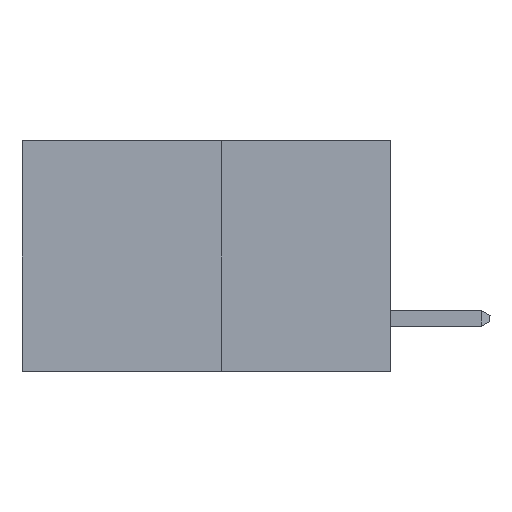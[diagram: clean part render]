
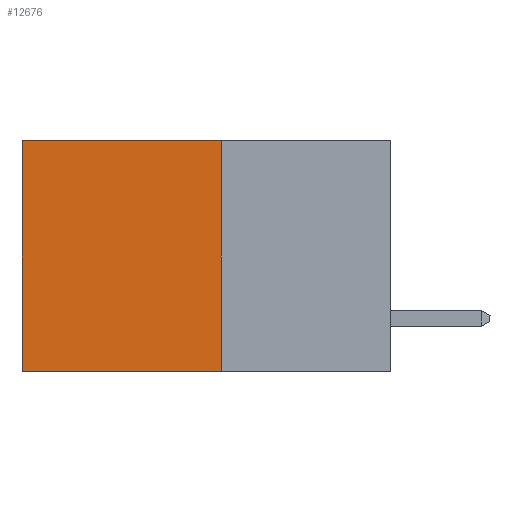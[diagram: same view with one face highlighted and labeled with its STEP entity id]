
A CAD part, left-side view. The second image highlights one B-rep face of the part: STEP entity #12676.
In plain terms, the highlighted planar face has unit normal (-1, 0, 0).
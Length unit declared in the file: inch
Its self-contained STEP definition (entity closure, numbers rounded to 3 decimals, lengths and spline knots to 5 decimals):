
#1009 = CARTESIAN_POINT ( 'NONE',  ( 0.277, 0.59, -0.37 ) ) ;
#1265 = VECTOR ( 'NONE', #9270, 39.37008 ) ;
#1685 = ORIENTED_EDGE ( 'NONE', *, *, #2820, .F. ) ;
#2820 = EDGE_CURVE ( 'NONE', #13778, #4900, #4460, .T. ) ;
#2873 = CARTESIAN_POINT ( 'NONE',  ( 0.277, 0.27, -0.37 ) ) ;
#2980 = DIRECTION ( 'NONE',  ( 0., 0., -1. ) ) ;
#3701 = LINE ( 'NONE', #12434, #9588 ) ;
#4460 = LINE ( 'NONE', #13301, #1265 ) ;
#4637 = EDGE_CURVE ( 'NONE', #13310, #13778, #6204, .T. ) ;
#4900 = VERTEX_POINT ( 'NONE', #1009 ) ;
#5039 = CARTESIAN_POINT ( 'NONE',  ( 0.277, 0.27, -0.37 ) ) ;
#5093 = DIRECTION ( 'NONE',  ( 0., 0., -1. ) ) ;
#5238 = ORIENTED_EDGE ( 'NONE', *, *, #4637, .F. ) ;
#5433 = VERTEX_POINT ( 'NONE', #12537 ) ;
#5515 = DIRECTION ( 'NONE',  ( 0., 0., -1. ) ) ;
#5531 = ORIENTED_EDGE ( 'NONE', *, *, #11087, .T. ) ;
#6204 = LINE ( 'NONE', #2873, #8958 ) ;
#6508 = ORIENTED_EDGE ( 'NONE', *, *, #9467, .T. ) ;
#7695 = CARTESIAN_POINT ( 'NONE',  ( 0.277, 0.27, 0. ) ) ;
#8197 = CARTESIAN_POINT ( 'NONE',  ( 0.277, 0.27, -0.37 ) ) ;
#8519 = FACE_OUTER_BOUND ( 'NONE', #14374, .T. ) ;
#8958 = VECTOR ( 'NONE', #2980, 39.37008 ) ;
#9270 = DIRECTION ( 'NONE',  ( 0., 1., 0. ) ) ;
#9467 = EDGE_CURVE ( 'NONE', #5433, #4900, #3701, .T. ) ;
#9588 = VECTOR ( 'NONE', #5515, 39.37008 ) ;
#9975 = LINE ( 'NONE', #10350, #14630 ) ;
#10350 = CARTESIAN_POINT ( 'NONE',  ( 0.277, 0.27, 0. ) ) ;
#10931 = PLANE ( 'NONE',  #13718 ) ;
#11087 = EDGE_CURVE ( 'NONE', #13310, #5433, #9975, .T. ) ;
#12044 = DIRECTION ( 'NONE',  ( 1., 0., 0. ) ) ;
#12434 = CARTESIAN_POINT ( 'NONE',  ( 0.277, 0.59, -0.37 ) ) ;
#12537 = CARTESIAN_POINT ( 'NONE',  ( 0.277, 0.59, 0. ) ) ;
#12676 = ADVANCED_FACE ( 'NONE', ( #8519 ), #10931, .F. ) ;
#13301 = CARTESIAN_POINT ( 'NONE',  ( 0.277, 0.27, -0.37 ) ) ;
#13310 = VERTEX_POINT ( 'NONE', #7695 ) ;
#13718 = AXIS2_PLACEMENT_3D ( 'NONE', #5039, #12044, #5093 ) ;
#13778 = VERTEX_POINT ( 'NONE', #8197 ) ;
#14374 = EDGE_LOOP ( 'NONE', ( #6508, #1685, #5238, #5531 ) ) ;
#14593 = DIRECTION ( 'NONE',  ( 0., 1., 0. ) ) ;
#14630 = VECTOR ( 'NONE', #14593, 39.37008 ) ;
